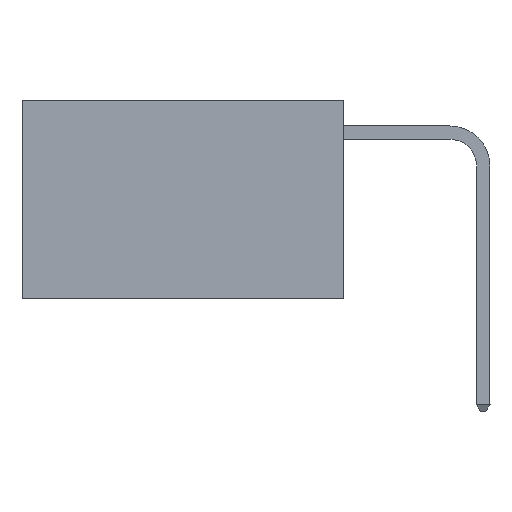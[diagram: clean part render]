
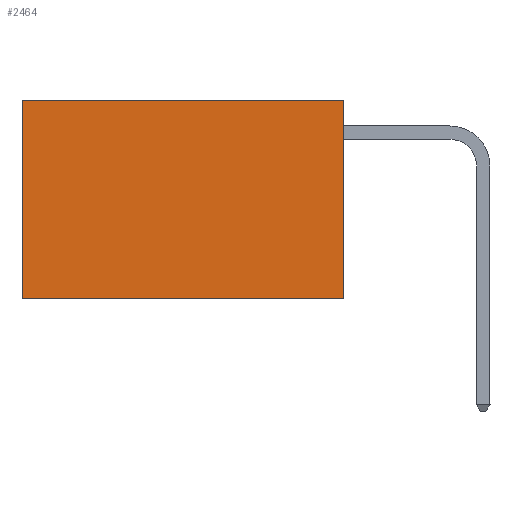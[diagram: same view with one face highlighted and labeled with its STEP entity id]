
A CAD part, left-side view. The second image highlights one B-rep face of the part: STEP entity #2464.
In plain terms, the highlighted planar face has unit normal (-1, 0, 0).
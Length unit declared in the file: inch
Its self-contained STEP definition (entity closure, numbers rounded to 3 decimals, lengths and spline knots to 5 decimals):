
#74 = VERTEX_POINT ( 'NONE', #4138 ) ;
#330 = EDGE_CURVE ( 'NONE', #5995, #74, #8391, .T. ) ;
#596 = LINE ( 'NONE', #3715, #9777 ) ;
#672 = CARTESIAN_POINT ( 'NONE',  ( 0.2625, 0.6, 0. ) ) ;
#978 = LINE ( 'NONE', #7443, #5643 ) ;
#1796 = DIRECTION ( 'NONE',  ( 0., 1., 0. ) ) ;
#1955 = DIRECTION ( 'NONE',  ( 0., 1., 0. ) ) ;
#2370 = CARTESIAN_POINT ( 'NONE',  ( 0.2625, 0., 0. ) ) ;
#2464 = ADVANCED_FACE ( 'NONE', ( #2707 ), #11458, .F. ) ;
#2707 = FACE_OUTER_BOUND ( 'NONE', #5459, .T. ) ;
#3124 = EDGE_CURVE ( 'NONE', #7999, #4776, #8754, .T. ) ;
#3378 = ORIENTED_EDGE ( 'NONE', *, *, #330, .F. ) ;
#3715 = CARTESIAN_POINT ( 'NONE',  ( 0.2625, 0.6, 0. ) ) ;
#4138 = CARTESIAN_POINT ( 'NONE',  ( 0.2625, 0.6, -0.37 ) ) ;
#4494 = CARTESIAN_POINT ( 'NONE',  ( 0.2625, 0., -0.37 ) ) ;
#4595 = DIRECTION ( 'NONE',  ( 0., 0., -1. ) ) ;
#4776 = VERTEX_POINT ( 'NONE', #672 ) ;
#5237 = CARTESIAN_POINT ( 'NONE',  ( 0.2625, 0., 0. ) ) ;
#5459 = EDGE_LOOP ( 'NONE', ( #6533, #3378, #8880, #9038 ) ) ;
#5643 = VECTOR ( 'NONE', #11049, 39.37008 ) ;
#5995 = VERTEX_POINT ( 'NONE', #7845 ) ;
#6367 = EDGE_CURVE ( 'NONE', #4776, #74, #596, .T. ) ;
#6533 = ORIENTED_EDGE ( 'NONE', *, *, #6367, .T. ) ;
#7443 = CARTESIAN_POINT ( 'NONE',  ( 0.2625, 0., 0. ) ) ;
#7481 = DIRECTION ( 'NONE',  ( 1., 0., 0. ) ) ;
#7538 = CARTESIAN_POINT ( 'NONE',  ( 0.2625, 0., 0. ) ) ;
#7845 = CARTESIAN_POINT ( 'NONE',  ( 0.2625, 0., -0.37 ) ) ;
#7988 = DIRECTION ( 'NONE',  ( 0., 0., -1. ) ) ;
#7999 = VERTEX_POINT ( 'NONE', #7538 ) ;
#8391 = LINE ( 'NONE', #4494, #10803 ) ;
#8594 = EDGE_CURVE ( 'NONE', #7999, #5995, #978, .T. ) ;
#8754 = LINE ( 'NONE', #5237, #10328 ) ;
#8880 = ORIENTED_EDGE ( 'NONE', *, *, #8594, .F. ) ;
#9038 = ORIENTED_EDGE ( 'NONE', *, *, #3124, .T. ) ;
#9777 = VECTOR ( 'NONE', #4595, 39.37008 ) ;
#10328 = VECTOR ( 'NONE', #1796, 39.37008 ) ;
#10541 = AXIS2_PLACEMENT_3D ( 'NONE', #2370, #7481, #7988 ) ;
#10803 = VECTOR ( 'NONE', #1955, 39.37008 ) ;
#11049 = DIRECTION ( 'NONE',  ( 0., 0., -1. ) ) ;
#11458 = PLANE ( 'NONE',  #10541 ) ;
